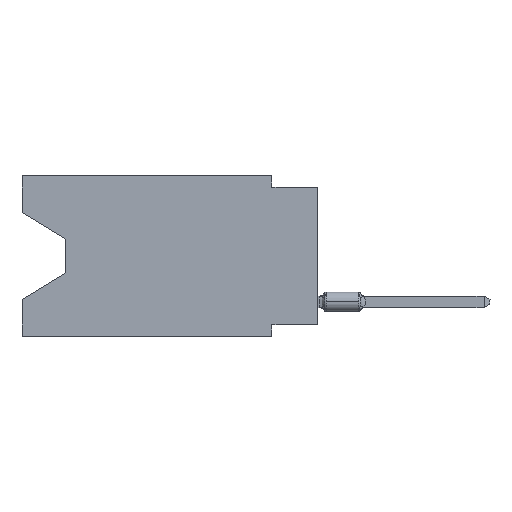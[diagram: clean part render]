
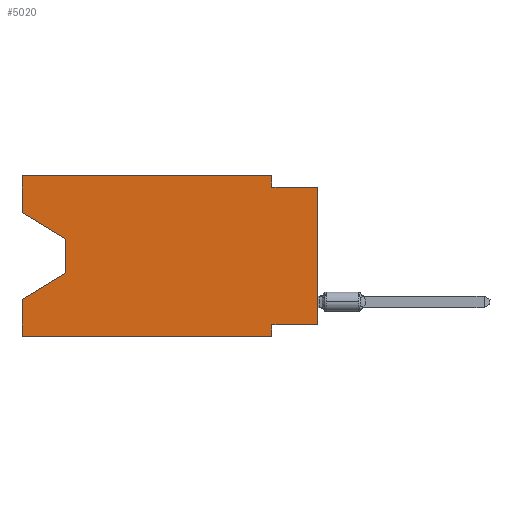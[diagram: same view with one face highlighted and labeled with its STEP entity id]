
A CAD part, left-side view. The second image highlights one B-rep face of the part: STEP entity #5020.
In plain terms, the highlighted planar face has unit normal (-1, 0, 0).
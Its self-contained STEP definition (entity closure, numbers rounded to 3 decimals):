
#74 = LINE ( 'NONE', #10496, #7013 ) ;
#98 = VERTEX_POINT ( 'NONE', #8346 ) ;
#151 = DIRECTION ( 'NONE',  ( 0., -0.855, -0.519 ) ) ;
#204 = DIRECTION ( 'NONE',  ( 0., 0., 1. ) ) ;
#328 = CARTESIAN_POINT ( 'NONE',  ( 0., 0., 0. ) ) ;
#390 = EDGE_CURVE ( 'NONE', #3164, #18085, #74, .T. ) ;
#572 = VERTEX_POINT ( 'NONE', #825 ) ;
#825 = CARTESIAN_POINT ( 'NONE',  ( 0., 2.54, -8.89 ) ) ;
#1251 = LINE ( 'NONE', #11770, #16902 ) ;
#1316 = VERTEX_POINT ( 'NONE', #4475 ) ;
#1467 = LINE ( 'NONE', #13453, #6998 ) ;
#1537 = LINE ( 'NONE', #328, #14832 ) ;
#1548 = DIRECTION ( 'NONE',  ( 0., 0., -1. ) ) ;
#1557 = LINE ( 'NONE', #15399, #15851 ) ;
#2313 = CARTESIAN_POINT ( 'NONE',  ( 0., 13.97, -3.505 ) ) ;
#3164 = VERTEX_POINT ( 'NONE', #17200 ) ;
#3332 = DIRECTION ( 'NONE',  ( 0., -1., 0. ) ) ;
#3403 = DIRECTION ( 'NONE',  ( 0., 0., -1. ) ) ;
#3503 = DIRECTION ( 'NONE',  ( 0., 0., 1. ) ) ;
#3655 = DIRECTION ( 'NONE',  ( 0., -1., 0. ) ) ;
#3702 = PLANE ( 'NONE',  #5138 ) ;
#4475 = CARTESIAN_POINT ( 'NONE',  ( 0., 16.383, -8.89 ) ) ;
#4656 = LINE ( 'NONE', #15348, #16099 ) ;
#4785 = EDGE_CURVE ( 'NONE', #14221, #572, #1251, .T. ) ;
#4955 = CARTESIAN_POINT ( 'NONE',  ( 0., 16.383, -6.852 ) ) ;
#5020 = ADVANCED_FACE ( 'NONE', ( #17151 ), #3702, .F. ) ;
#5138 = AXIS2_PLACEMENT_3D ( 'NONE', #9694, #6940, #5559 ) ;
#5383 = ORIENTED_EDGE ( 'NONE', *, *, #8958, .T. ) ;
#5409 = VECTOR ( 'NONE', #204, 1000. ) ;
#5536 = LINE ( 'NONE', #8218, #9816 ) ;
#5559 = DIRECTION ( 'NONE',  ( 0., 0., -1. ) ) ;
#6067 = ORIENTED_EDGE ( 'NONE', *, *, #4785, .F. ) ;
#6841 = ORIENTED_EDGE ( 'NONE', *, *, #15331, .T. ) ;
#6940 = DIRECTION ( 'NONE',  ( 1., 0., 0. ) ) ;
#6998 = VECTOR ( 'NONE', #3332, 1000. ) ;
#7013 = VECTOR ( 'NONE', #9470, 1000. ) ;
#7300 = ORIENTED_EDGE ( 'NONE', *, *, #10050, .F. ) ;
#7558 = DIRECTION ( 'NONE',  ( 0., -1., 0. ) ) ;
#7954 = CARTESIAN_POINT ( 'NONE',  ( 0., 16.383, -2.038 ) ) ;
#8218 = CARTESIAN_POINT ( 'NONE',  ( 0., 2.54, 0. ) ) ;
#8346 = CARTESIAN_POINT ( 'NONE',  ( 0., 2.54, -0.635 ) ) ;
#8958 = EDGE_CURVE ( 'NONE', #18825, #15533, #17733, .T. ) ;
#8975 = DIRECTION ( 'NONE',  ( 0., 1., 0. ) ) ;
#8996 = CARTESIAN_POINT ( 'NONE',  ( 0., 16.383, -2.038 ) ) ;
#9297 = CARTESIAN_POINT ( 'NONE',  ( 0., 16.383, 0. ) ) ;
#9470 = DIRECTION ( 'NONE',  ( 0., 0.855, -0.519 ) ) ;
#9525 = ORIENTED_EDGE ( 'NONE', *, *, #14844, .F. ) ;
#9694 = CARTESIAN_POINT ( 'NONE',  ( 0., 16.383, 0. ) ) ;
#9718 = CARTESIAN_POINT ( 'NONE',  ( 0., 2.54, 0. ) ) ;
#9816 = VECTOR ( 'NONE', #11518, 1000. ) ;
#9832 = VERTEX_POINT ( 'NONE', #12608 ) ;
#9858 = ORIENTED_EDGE ( 'NONE', *, *, #11684, .F. ) ;
#9904 = ORIENTED_EDGE ( 'NONE', *, *, #19404, .F. ) ;
#10050 = EDGE_CURVE ( 'NONE', #14075, #14221, #4656, .T. ) ;
#10241 = EDGE_CURVE ( 'NONE', #98, #9832, #15638, .T. ) ;
#10496 = CARTESIAN_POINT ( 'NONE',  ( 0., 13.97, -5.385 ) ) ;
#11024 = CARTESIAN_POINT ( 'NONE',  ( 0., 0., -0.635 ) ) ;
#11223 = ORIENTED_EDGE ( 'NONE', *, *, #10241, .F. ) ;
#11306 = CARTESIAN_POINT ( 'NONE',  ( 0., 2.54, -8.255 ) ) ;
#11518 = DIRECTION ( 'NONE',  ( 0., 0., -1. ) ) ;
#11684 = EDGE_CURVE ( 'NONE', #18825, #13396, #18369, .T. ) ;
#11770 = CARTESIAN_POINT ( 'NONE',  ( 0., 2.54, -8.89 ) ) ;
#12173 = EDGE_CURVE ( 'NONE', #1316, #572, #1467, .T. ) ;
#12310 = DIRECTION ( 'NONE',  ( 0., 0., 1. ) ) ;
#12548 = EDGE_CURVE ( 'NONE', #14075, #9832, #1537, .T. ) ;
#12608 = CARTESIAN_POINT ( 'NONE',  ( 0., 0., -0.635 ) ) ;
#12922 = VERTEX_POINT ( 'NONE', #9718 ) ;
#13359 = VECTOR ( 'NONE', #3403, 1000. ) ;
#13396 = VERTEX_POINT ( 'NONE', #18737 ) ;
#13453 = CARTESIAN_POINT ( 'NONE',  ( 0., 16.383, -8.89 ) ) ;
#13708 = CARTESIAN_POINT ( 'NONE',  ( 0., 0., -8.255 ) ) ;
#14075 = VERTEX_POINT ( 'NONE', #13708 ) ;
#14221 = VERTEX_POINT ( 'NONE', #11306 ) ;
#14600 = EDGE_LOOP ( 'NONE', ( #5383, #6841, #18084, #18816, #17619, #6067, #7300, #15600, #11223, #9904, #9525, #9858 ) ) ;
#14832 = VECTOR ( 'NONE', #12310, 1000. ) ;
#14844 = EDGE_CURVE ( 'NONE', #13396, #12922, #1557, .T. ) ;
#14883 = VECTOR ( 'NONE', #3503, 1000. ) ;
#15323 = CARTESIAN_POINT ( 'NONE',  ( 0., 16.383, 0. ) ) ;
#15331 = EDGE_CURVE ( 'NONE', #15533, #3164, #15570, .T. ) ;
#15348 = CARTESIAN_POINT ( 'NONE',  ( 0., 0., -8.255 ) ) ;
#15399 = CARTESIAN_POINT ( 'NONE',  ( 0., 16.383, 0. ) ) ;
#15533 = VERTEX_POINT ( 'NONE', #15958 ) ;
#15570 = LINE ( 'NONE', #2313, #13359 ) ;
#15578 = LINE ( 'NONE', #9297, #14883 ) ;
#15600 = ORIENTED_EDGE ( 'NONE', *, *, #12548, .T. ) ;
#15638 = LINE ( 'NONE', #11024, #18295 ) ;
#15851 = VECTOR ( 'NONE', #7558, 1000. ) ;
#15958 = CARTESIAN_POINT ( 'NONE',  ( 0., 13.97, -3.505 ) ) ;
#16099 = VECTOR ( 'NONE', #8975, 1000. ) ;
#16684 = VECTOR ( 'NONE', #151, 1000. ) ;
#16902 = VECTOR ( 'NONE', #1548, 1000. ) ;
#17151 = FACE_OUTER_BOUND ( 'NONE', #14600, .T. ) ;
#17200 = CARTESIAN_POINT ( 'NONE',  ( 0., 13.97, -5.385 ) ) ;
#17619 = ORIENTED_EDGE ( 'NONE', *, *, #12173, .T. ) ;
#17660 = EDGE_CURVE ( 'NONE', #1316, #18085, #15578, .T. ) ;
#17733 = LINE ( 'NONE', #8996, #16684 ) ;
#18084 = ORIENTED_EDGE ( 'NONE', *, *, #390, .T. ) ;
#18085 = VERTEX_POINT ( 'NONE', #4955 ) ;
#18295 = VECTOR ( 'NONE', #3655, 1000. ) ;
#18369 = LINE ( 'NONE', #15323, #5409 ) ;
#18737 = CARTESIAN_POINT ( 'NONE',  ( 0., 16.383, 0. ) ) ;
#18816 = ORIENTED_EDGE ( 'NONE', *, *, #17660, .F. ) ;
#18825 = VERTEX_POINT ( 'NONE', #7954 ) ;
#19404 = EDGE_CURVE ( 'NONE', #12922, #98, #5536, .T. ) ;
